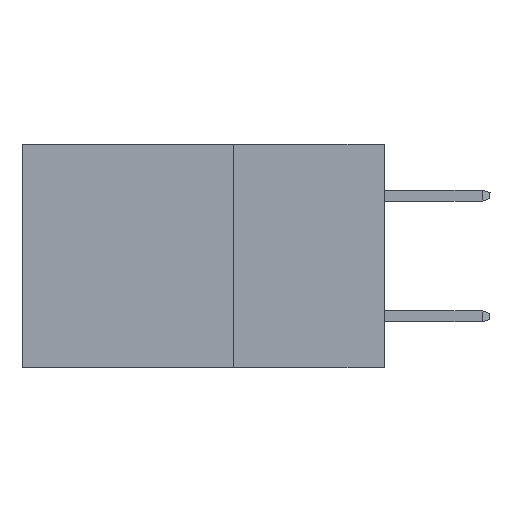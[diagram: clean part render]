
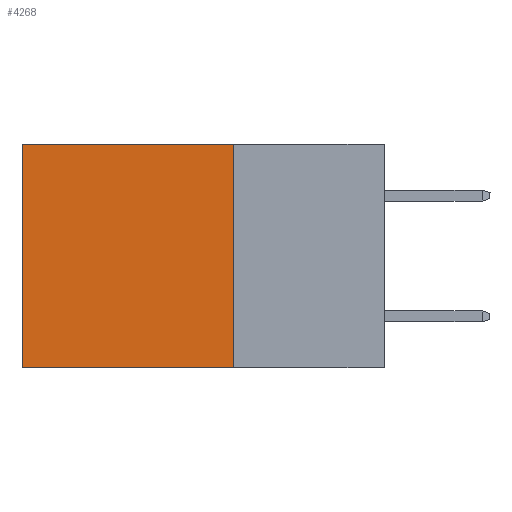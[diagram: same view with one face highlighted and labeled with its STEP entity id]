
A CAD part, left-side view. The second image highlights one B-rep face of the part: STEP entity #4268.
In plain terms, the highlighted planar face has unit normal (-1, 0, 0).
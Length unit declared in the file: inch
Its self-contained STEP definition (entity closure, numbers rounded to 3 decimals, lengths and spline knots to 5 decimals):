
#715 = CARTESIAN_POINT ( 'NONE',  ( 0.298, 0.25, -0.37 ) ) ;
#737 = CARTESIAN_POINT ( 'NONE',  ( 0.298, 0.6, 0. ) ) ;
#942 = CARTESIAN_POINT ( 'NONE',  ( 0.298, 0.6, -0.37 ) ) ;
#1094 = DIRECTION ( 'NONE',  ( 0., 1., 0. ) ) ;
#1312 = ORIENTED_EDGE ( 'NONE', *, *, #2717, .F. ) ;
#1644 = EDGE_LOOP ( 'NONE', ( #13100, #6697, #1312, #4100 ) ) ;
#2198 = PLANE ( 'NONE',  #9304 ) ;
#2717 = EDGE_CURVE ( 'NONE', #13482, #4464, #9284, .T. ) ;
#3010 = CARTESIAN_POINT ( 'NONE',  ( 0.298, 0.6, 0. ) ) ;
#3021 = DIRECTION ( 'NONE',  ( 0., 0., -1. ) ) ;
#3217 = DIRECTION ( 'NONE',  ( 0., 0., -1. ) ) ;
#3670 = VECTOR ( 'NONE', #1094, 39.37008 ) ;
#3789 = VERTEX_POINT ( 'NONE', #3010 ) ;
#4100 = ORIENTED_EDGE ( 'NONE', *, *, #4736, .T. ) ;
#4268 = ADVANCED_FACE ( 'NONE', ( #13166 ), #2198, .F. ) ;
#4448 = EDGE_CURVE ( 'NONE', #3789, #12957, #7357, .T. ) ;
#4464 = VERTEX_POINT ( 'NONE', #10866 ) ;
#4559 = LINE ( 'NONE', #7811, #3670 ) ;
#4736 = EDGE_CURVE ( 'NONE', #13482, #3789, #4559, .T. ) ;
#5409 = VECTOR ( 'NONE', #5952, 39.37008 ) ;
#5659 = CARTESIAN_POINT ( 'NONE',  ( 0.298, 0.25, 0. ) ) ;
#5952 = DIRECTION ( 'NONE',  ( 0., 0., -1. ) ) ;
#6697 = ORIENTED_EDGE ( 'NONE', *, *, #11953, .F. ) ;
#7324 = LINE ( 'NONE', #715, #10517 ) ;
#7357 = LINE ( 'NONE', #737, #10017 ) ;
#7811 = CARTESIAN_POINT ( 'NONE',  ( 0.298, 0.25, 0. ) ) ;
#8809 = DIRECTION ( 'NONE',  ( 1., 0., 0. ) ) ;
#9284 = LINE ( 'NONE', #10537, #5409 ) ;
#9304 = AXIS2_PLACEMENT_3D ( 'NONE', #14396, #8809, #3217 ) ;
#10017 = VECTOR ( 'NONE', #3021, 39.37008 ) ;
#10517 = VECTOR ( 'NONE', #11907, 39.37008 ) ;
#10537 = CARTESIAN_POINT ( 'NONE',  ( 0.298, 0.25, 0. ) ) ;
#10866 = CARTESIAN_POINT ( 'NONE',  ( 0.298, 0.25, -0.37 ) ) ;
#11907 = DIRECTION ( 'NONE',  ( 0., 1., 0. ) ) ;
#11953 = EDGE_CURVE ( 'NONE', #4464, #12957, #7324, .T. ) ;
#12957 = VERTEX_POINT ( 'NONE', #942 ) ;
#13100 = ORIENTED_EDGE ( 'NONE', *, *, #4448, .T. ) ;
#13166 = FACE_OUTER_BOUND ( 'NONE', #1644, .T. ) ;
#13482 = VERTEX_POINT ( 'NONE', #5659 ) ;
#14396 = CARTESIAN_POINT ( 'NONE',  ( 0.298, 0.25, 0. ) ) ;
